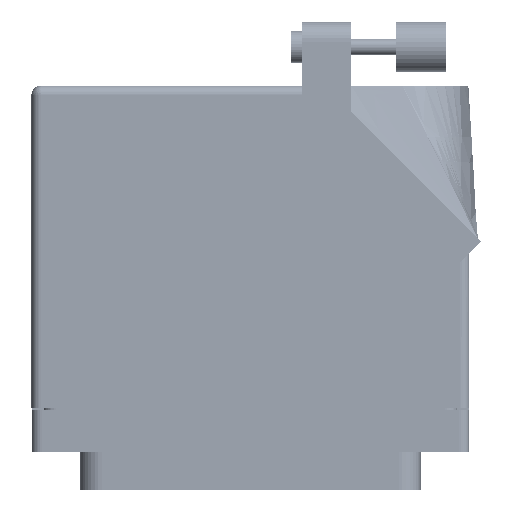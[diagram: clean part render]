
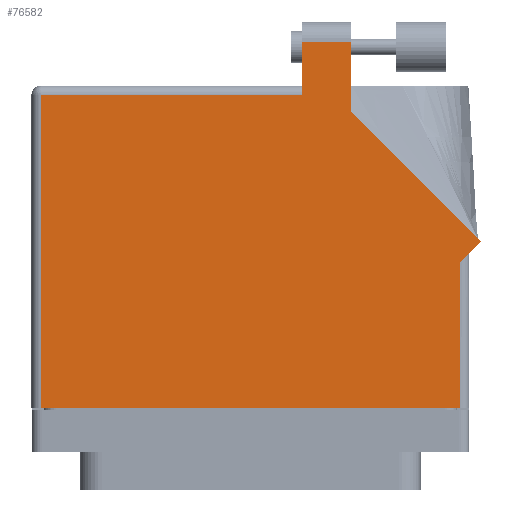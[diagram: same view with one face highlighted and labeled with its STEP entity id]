
A CAD part, front view. The second image highlights one B-rep face of the part: STEP entity #76582.
In plain terms, the highlighted face is planar.
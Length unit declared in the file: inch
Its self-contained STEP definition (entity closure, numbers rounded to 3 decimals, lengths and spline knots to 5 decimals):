
#563 = LINE ( 'NONE', #51189, #37190 ) ;
#677 = VERTEX_POINT ( 'NONE', #48179 ) ;
#2714 = CARTESIAN_POINT ( 'NONE',  ( 1.3155, -0.1, 0.765 ) ) ;
#3665 = ORIENTED_EDGE ( 'NONE', *, *, #4423, .T. ) ;
#3847 = ORIENTED_EDGE ( 'NONE', *, *, #39506, .T. ) ;
#4423 = EDGE_CURVE ( 'NONE', #11121, #677, #17456, .T. ) ;
#4654 = VECTOR ( 'NONE', #57199, 39.37008 ) ;
#7608 = LINE ( 'NONE', #22435, #60440 ) ;
#7787 = PLANE ( 'NONE',  #31496 ) ;
#9093 = EDGE_CURVE ( 'NONE', #73650, #49694, #66617, .T. ) ;
#9211 = VERTEX_POINT ( 'NONE', #71065 ) ;
#9336 = EDGE_CURVE ( 'NONE', #49694, #88900, #50302, .T. ) ;
#9366 = VECTOR ( 'NONE', #11127, 39.37008 ) ;
#9624 = CARTESIAN_POINT ( 'NONE',  ( -1.3155, 1.868, 0.765 ) ) ;
#10660 = EDGE_CURVE ( 'NONE', #22488, #9211, #23098, .T. ) ;
#10706 = DIRECTION ( 'NONE',  ( 0., -1., 0. ) ) ;
#11121 = VERTEX_POINT ( 'NONE', #15233 ) ;
#11127 = DIRECTION ( 'NONE',  ( -1., 0., 0. ) ) ;
#11431 = CARTESIAN_POINT ( 'NONE',  ( 0.3275, 2.205, 0.765 ) ) ;
#15233 = CARTESIAN_POINT ( 'NONE',  ( 1.3155, 0.818, 0.765 ) ) ;
#15586 = CARTESIAN_POINT ( 'NONE',  ( 0.3275, 1.868, 0.765 ) ) ;
#17456 = LINE ( 'NONE', #29579, #49733 ) ;
#20439 = CARTESIAN_POINT ( 'NONE',  ( -1.3155, -0.1, 0.765 ) ) ;
#22435 = CARTESIAN_POINT ( 'NONE',  ( -1.3775, 1.868, 0.765 ) ) ;
#22488 = VERTEX_POINT ( 'NONE', #9624 ) ;
#23098 = LINE ( 'NONE', #20439, #45768 ) ;
#23226 = EDGE_CURVE ( 'NONE', #88900, #22488, #7608, .T. ) ;
#24176 = DIRECTION ( 'NONE',  ( 0.707, 0.707, 0. ) ) ;
#24231 = ORIENTED_EDGE ( 'NONE', *, *, #9336, .T. ) ;
#26364 = ORIENTED_EDGE ( 'NONE', *, *, #39333, .T. ) ;
#26707 = EDGE_CURVE ( 'NONE', #32374, #73650, #563, .T. ) ;
#28306 = ORIENTED_EDGE ( 'NONE', *, *, #10660, .T. ) ;
#29579 = CARTESIAN_POINT ( 'NONE',  ( 1.3775, 0.88, 0.765 ) ) ;
#29714 = DIRECTION ( 'NONE',  ( 0., 0., -1. ) ) ;
#31496 = AXIS2_PLACEMENT_3D ( 'NONE', #64108, #29714, #55963 ) ;
#32374 = VERTEX_POINT ( 'NONE', #68259 ) ;
#32618 = LINE ( 'NONE', #59643, #72623 ) ;
#33482 = LINE ( 'NONE', #88301, #51904 ) ;
#36914 = EDGE_LOOP ( 'NONE', ( #76076, #54164, #24231, #40345, #28306, #3847, #26364, #3665, #51605 ) ) ;
#37190 = VECTOR ( 'NONE', #57491, 39.37008 ) ;
#39333 = EDGE_CURVE ( 'NONE', #44029, #11121, #32618, .T. ) ;
#39506 = EDGE_CURVE ( 'NONE', #9211, #44029, #52084, .T. ) ;
#40345 = ORIENTED_EDGE ( 'NONE', *, *, #23226, .T. ) ;
#44029 = VERTEX_POINT ( 'NONE', #2714 ) ;
#45768 = VECTOR ( 'NONE', #82281, 39.37008 ) ;
#48179 = CARTESIAN_POINT ( 'NONE',  ( 1.44821, 0.95071, 0.765 ) ) ;
#49694 = VERTEX_POINT ( 'NONE', #73686 ) ;
#49733 = VECTOR ( 'NONE', #24176, 39.37008 ) ;
#50302 = LINE ( 'NONE', #72589, #55651 ) ;
#51189 = CARTESIAN_POINT ( 'NONE',  ( 0.6345, 1.76442, 0.765 ) ) ;
#51605 = ORIENTED_EDGE ( 'NONE', *, *, #65426, .T. ) ;
#51904 = VECTOR ( 'NONE', #60757, 39.37008 ) ;
#52084 = LINE ( 'NONE', #63893, #4654 ) ;
#52761 = DIRECTION ( 'NONE',  ( 0., 1., 0. ) ) ;
#54164 = ORIENTED_EDGE ( 'NONE', *, *, #9093, .T. ) ;
#55651 = VECTOR ( 'NONE', #10706, 39.37008 ) ;
#55963 = DIRECTION ( 'NONE',  ( -1., 0., 0. ) ) ;
#56585 = CARTESIAN_POINT ( 'NONE',  ( 0.6345, 2.205, 0.765 ) ) ;
#57199 = DIRECTION ( 'NONE',  ( 1., 0., 0. ) ) ;
#57491 = DIRECTION ( 'NONE',  ( 0., 1., 0. ) ) ;
#59643 = CARTESIAN_POINT ( 'NONE',  ( 1.3155, 0.88, 0.765 ) ) ;
#60440 = VECTOR ( 'NONE', #84575, 39.37008 ) ;
#60757 = DIRECTION ( 'NONE',  ( -0.707, 0.707, 0. ) ) ;
#63893 = CARTESIAN_POINT ( 'NONE',  ( -1.3775, -0.1, 0.765 ) ) ;
#64108 = CARTESIAN_POINT ( 'NONE',  ( -1.3775, 1.93, 0.765 ) ) ;
#65426 = EDGE_CURVE ( 'NONE', #677, #32374, #33482, .T. ) ;
#66617 = LINE ( 'NONE', #11431, #9366 ) ;
#68259 = CARTESIAN_POINT ( 'NONE',  ( 0.6345, 1.76442, 0.765 ) ) ;
#71065 = CARTESIAN_POINT ( 'NONE',  ( -1.3155, -0.1, 0.765 ) ) ;
#72589 = CARTESIAN_POINT ( 'NONE',  ( 0.3275, 1.93, 0.765 ) ) ;
#72623 = VECTOR ( 'NONE', #52761, 39.37008 ) ;
#73650 = VERTEX_POINT ( 'NONE', #56585 ) ;
#73686 = CARTESIAN_POINT ( 'NONE',  ( 0.3275, 2.205, 0.765 ) ) ;
#76076 = ORIENTED_EDGE ( 'NONE', *, *, #26707, .T. ) ;
#76582 = ADVANCED_FACE ( 'NONE', ( #82294 ), #7787, .F. ) ;
#82281 = DIRECTION ( 'NONE',  ( 0., -1., 0. ) ) ;
#82294 = FACE_OUTER_BOUND ( 'NONE', #36914, .T. ) ;
#84575 = DIRECTION ( 'NONE',  ( -1., 0., 0. ) ) ;
#88301 = CARTESIAN_POINT ( 'NONE',  ( 1.44821, 0.95071, 0.765 ) ) ;
#88900 = VERTEX_POINT ( 'NONE', #15586 ) ;
